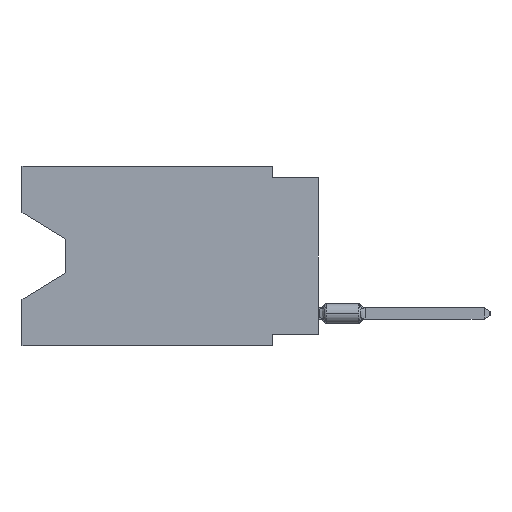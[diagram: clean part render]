
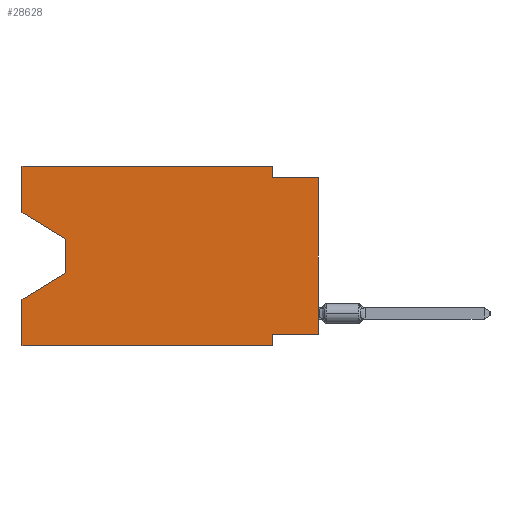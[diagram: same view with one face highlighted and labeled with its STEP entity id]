
A CAD part, left-side view. The second image highlights one B-rep face of the part: STEP entity #28628.
In plain terms, the highlighted planar face has unit normal (-1, 0, 0).
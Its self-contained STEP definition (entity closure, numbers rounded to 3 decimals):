
#161 = DIRECTION ( 'NONE',  ( 0., 0.855, -0.519 ) ) ;
#538 = LINE ( 'NONE', #43066, #46877 ) ;
#1003 = VERTEX_POINT ( 'NONE', #7135 ) ;
#1180 = ORIENTED_EDGE ( 'NONE', *, *, #40466, .F. ) ;
#3429 = DIRECTION ( 'NONE',  ( 0., 0., 1. ) ) ;
#4029 = ORIENTED_EDGE ( 'NONE', *, *, #51960, .F. ) ;
#4557 = DIRECTION ( 'NONE',  ( 0., -1., 0. ) ) ;
#5991 = ORIENTED_EDGE ( 'NONE', *, *, #65976, .F. ) ;
#7135 = CARTESIAN_POINT ( 'NONE',  ( 0., 2.54, 0. ) ) ;
#8595 = ORIENTED_EDGE ( 'NONE', *, *, #27983, .T. ) ;
#9405 = PLANE ( 'NONE',  #41681 ) ;
#10340 = CARTESIAN_POINT ( 'NONE',  ( 0., 0., 0. ) ) ;
#11032 = CARTESIAN_POINT ( 'NONE',  ( 0., 16.383, -9.906 ) ) ;
#11713 = VERTEX_POINT ( 'NONE', #11032 ) ;
#11747 = VECTOR ( 'NONE', #3429, 1000. ) ;
#13320 = CARTESIAN_POINT ( 'NONE',  ( 0., 16.383, 0. ) ) ;
#14198 = CARTESIAN_POINT ( 'NONE',  ( 0., 13.97, -5.893 ) ) ;
#14784 = DIRECTION ( 'NONE',  ( 0., 0., -1. ) ) ;
#15120 = LINE ( 'NONE', #39248, #37232 ) ;
#15603 = CARTESIAN_POINT ( 'NONE',  ( 0., 16.383, 0. ) ) ;
#15985 = EDGE_CURVE ( 'NONE', #29505, #53614, #63426, .T. ) ;
#17808 = LINE ( 'NONE', #45414, #21898 ) ;
#18192 = VERTEX_POINT ( 'NONE', #15603 ) ;
#18583 = ORIENTED_EDGE ( 'NONE', *, *, #52673, .F. ) ;
#21533 = DIRECTION ( 'NONE',  ( 0., -1., 0. ) ) ;
#21898 = VECTOR ( 'NONE', #161, 1000. ) ;
#22692 = VERTEX_POINT ( 'NONE', #37652 ) ;
#22804 = VERTEX_POINT ( 'NONE', #29092 ) ;
#23357 = ORIENTED_EDGE ( 'NONE', *, *, #46038, .F. ) ;
#23687 = EDGE_CURVE ( 'NONE', #53614, #22804, #17808, .T. ) ;
#24360 = VERTEX_POINT ( 'NONE', #48730 ) ;
#25800 = VECTOR ( 'NONE', #75306, 1000. ) ;
#26449 = DIRECTION ( 'NONE',  ( 0., 0., -1. ) ) ;
#26573 = ORIENTED_EDGE ( 'NONE', *, *, #23687, .T. ) ;
#26889 = LINE ( 'NONE', #67909, #67608 ) ;
#27205 = CARTESIAN_POINT ( 'NONE',  ( 0., 2.54, -9.906 ) ) ;
#27936 = CARTESIAN_POINT ( 'NONE',  ( 0., 2.54, 0. ) ) ;
#27983 = EDGE_CURVE ( 'NONE', #24360, #50955, #63237, .T. ) ;
#28628 = ADVANCED_FACE ( 'NONE', ( #37765 ), #9405, .F. ) ;
#29092 = CARTESIAN_POINT ( 'NONE',  ( 0., 16.383, -7.36 ) ) ;
#29505 = VERTEX_POINT ( 'NONE', #56584 ) ;
#30180 = DIRECTION ( 'NONE',  ( 0., 0., 1. ) ) ;
#30329 = ORIENTED_EDGE ( 'NONE', *, *, #43991, .F. ) ;
#30898 = ORIENTED_EDGE ( 'NONE', *, *, #60466, .T. ) ;
#31870 = VERTEX_POINT ( 'NONE', #65562 ) ;
#32187 = CARTESIAN_POINT ( 'NONE',  ( 0., 16.383, 0. ) ) ;
#33858 = LINE ( 'NONE', #63768, #45273 ) ;
#36846 = CARTESIAN_POINT ( 'NONE',  ( 0., 16.383, -2.546 ) ) ;
#37232 = VECTOR ( 'NONE', #38485, 1000. ) ;
#37652 = CARTESIAN_POINT ( 'NONE',  ( 0., 2.54, -0.635 ) ) ;
#37765 = FACE_OUTER_BOUND ( 'NONE', #42697, .T. ) ;
#38485 = DIRECTION ( 'NONE',  ( 0., -0.855, -0.519 ) ) ;
#39248 = CARTESIAN_POINT ( 'NONE',  ( 0., 16.383, -2.546 ) ) ;
#39451 = CARTESIAN_POINT ( 'NONE',  ( 0., 16.383, -9.906 ) ) ;
#40466 = EDGE_CURVE ( 'NONE', #22692, #50955, #26889, .T. ) ;
#41681 = AXIS2_PLACEMENT_3D ( 'NONE', #43901, #60802, #14784 ) ;
#42697 = EDGE_LOOP ( 'NONE', ( #30898, #58088, #26573, #4029, #47676, #23357, #5991, #8595, #1180, #18583, #43632, #30329 ) ) ;
#43066 = CARTESIAN_POINT ( 'NONE',  ( 0., 0., -9.271 ) ) ;
#43390 = VERTEX_POINT ( 'NONE', #52901 ) ;
#43632 = ORIENTED_EDGE ( 'NONE', *, *, #44690, .F. ) ;
#43901 = CARTESIAN_POINT ( 'NONE',  ( 0., 16.383, 0. ) ) ;
#43912 = VECTOR ( 'NONE', #30180, 1000. ) ;
#43991 = EDGE_CURVE ( 'NONE', #57326, #18192, #70445, .T. ) ;
#44690 = EDGE_CURVE ( 'NONE', #18192, #1003, #33858, .T. ) ;
#45273 = VECTOR ( 'NONE', #74130, 1000. ) ;
#45414 = CARTESIAN_POINT ( 'NONE',  ( 0., 13.97, -5.893 ) ) ;
#45950 = DIRECTION ( 'NONE',  ( 0., 0., -1. ) ) ;
#46038 = EDGE_CURVE ( 'NONE', #43390, #31870, #49466, .T. ) ;
#46877 = VECTOR ( 'NONE', #48439, 1000. ) ;
#47676 = ORIENTED_EDGE ( 'NONE', *, *, #61304, .T. ) ;
#48439 = DIRECTION ( 'NONE',  ( 0., 1., 0. ) ) ;
#48730 = CARTESIAN_POINT ( 'NONE',  ( 0., 0., -9.271 ) ) ;
#49466 = LINE ( 'NONE', #27205, #58860 ) ;
#50955 = VERTEX_POINT ( 'NONE', #58494 ) ;
#51960 = EDGE_CURVE ( 'NONE', #11713, #22804, #66716, .T. ) ;
#52673 = EDGE_CURVE ( 'NONE', #1003, #22692, #63572, .T. ) ;
#52901 = CARTESIAN_POINT ( 'NONE',  ( 0., 2.54, -9.271 ) ) ;
#53614 = VERTEX_POINT ( 'NONE', #14198 ) ;
#53805 = VECTOR ( 'NONE', #75485, 1000. ) ;
#56584 = CARTESIAN_POINT ( 'NONE',  ( 0., 13.97, -4.013 ) ) ;
#57326 = VERTEX_POINT ( 'NONE', #36846 ) ;
#57448 = LINE ( 'NONE', #39451, #70389 ) ;
#57683 = CARTESIAN_POINT ( 'NONE',  ( 0., 13.97, -4.013 ) ) ;
#58088 = ORIENTED_EDGE ( 'NONE', *, *, #15985, .T. ) ;
#58494 = CARTESIAN_POINT ( 'NONE',  ( 0., 0., -0.635 ) ) ;
#58860 = VECTOR ( 'NONE', #26449, 1000. ) ;
#60466 = EDGE_CURVE ( 'NONE', #57326, #29505, #15120, .T. ) ;
#60802 = DIRECTION ( 'NONE',  ( 1., 0., 0. ) ) ;
#61304 = EDGE_CURVE ( 'NONE', #11713, #31870, #57448, .T. ) ;
#63237 = LINE ( 'NONE', #10340, #53805 ) ;
#63426 = LINE ( 'NONE', #57683, #25800 ) ;
#63572 = LINE ( 'NONE', #27936, #65985 ) ;
#63768 = CARTESIAN_POINT ( 'NONE',  ( 0., 16.383, 0. ) ) ;
#65562 = CARTESIAN_POINT ( 'NONE',  ( 0., 2.54, -9.906 ) ) ;
#65976 = EDGE_CURVE ( 'NONE', #24360, #43390, #538, .T. ) ;
#65985 = VECTOR ( 'NONE', #45950, 1000. ) ;
#66716 = LINE ( 'NONE', #32187, #11747 ) ;
#67608 = VECTOR ( 'NONE', #21533, 1000. ) ;
#67909 = CARTESIAN_POINT ( 'NONE',  ( 0., 0., -0.635 ) ) ;
#70389 = VECTOR ( 'NONE', #4557, 1000. ) ;
#70445 = LINE ( 'NONE', #13320, #43912 ) ;
#74130 = DIRECTION ( 'NONE',  ( 0., -1., 0. ) ) ;
#75306 = DIRECTION ( 'NONE',  ( 0., 0., -1. ) ) ;
#75485 = DIRECTION ( 'NONE',  ( 0., 0., 1. ) ) ;
